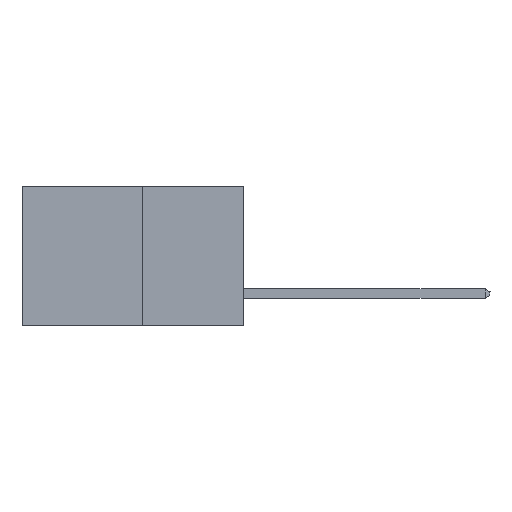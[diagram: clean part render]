
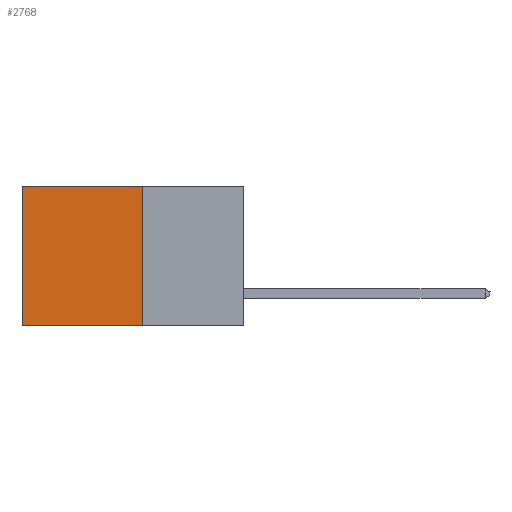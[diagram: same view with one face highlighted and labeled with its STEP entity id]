
A CAD part, left-side view. The second image highlights one B-rep face of the part: STEP entity #2768.
In plain terms, the highlighted planar face has unit normal (-1, 0, 0).
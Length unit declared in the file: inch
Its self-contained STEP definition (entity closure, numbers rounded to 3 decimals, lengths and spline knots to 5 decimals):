
#472 = CARTESIAN_POINT ( 'NONE',  ( 0.277, 0.27, -0.37 ) ) ;
#800 = VERTEX_POINT ( 'NONE', #4747 ) ;
#2022 = EDGE_CURVE ( 'NONE', #10014, #5146, #2332, .T. ) ;
#2332 = LINE ( 'NONE', #14295, #5473 ) ;
#2768 = ADVANCED_FACE ( 'NONE', ( #7432 ), #4299, .F. ) ;
#2903 = EDGE_LOOP ( 'NONE', ( #13023, #15455, #13230, #13313 ) ) ;
#4299 = PLANE ( 'NONE',  #10440 ) ;
#4747 = CARTESIAN_POINT ( 'NONE',  ( 0.277, 0.59, -0.37 ) ) ;
#4897 = VECTOR ( 'NONE', #15755, 39.37008 ) ;
#5146 = VERTEX_POINT ( 'NONE', #472 ) ;
#5473 = VECTOR ( 'NONE', #13830, 39.37008 ) ;
#5757 = DIRECTION ( 'NONE',  ( 0., 1., 0. ) ) ;
#7432 = FACE_OUTER_BOUND ( 'NONE', #2903, .T. ) ;
#7730 = VECTOR ( 'NONE', #16216, 39.37008 ) ;
#9906 = CARTESIAN_POINT ( 'NONE',  ( 0.277, 0.27, 0. ) ) ;
#10014 = VERTEX_POINT ( 'NONE', #14339 ) ;
#10440 = AXIS2_PLACEMENT_3D ( 'NONE', #14002, #14050, #14364 ) ;
#11548 = LINE ( 'NONE', #9906, #4897 ) ;
#12182 = LINE ( 'NONE', #12726, #7730 ) ;
#12311 = VECTOR ( 'NONE', #5757, 39.37008 ) ;
#12726 = CARTESIAN_POINT ( 'NONE',  ( 0.277, 0.59, -0.37 ) ) ;
#13023 = ORIENTED_EDGE ( 'NONE', *, *, #13631, .T. ) ;
#13230 = ORIENTED_EDGE ( 'NONE', *, *, #2022, .F. ) ;
#13313 = ORIENTED_EDGE ( 'NONE', *, *, #15853, .T. ) ;
#13631 = EDGE_CURVE ( 'NONE', #14796, #800, #12182, .T. ) ;
#13830 = DIRECTION ( 'NONE',  ( 0., 0., -1. ) ) ;
#14002 = CARTESIAN_POINT ( 'NONE',  ( 0.277, 0.27, -0.37 ) ) ;
#14050 = DIRECTION ( 'NONE',  ( 1., 0., 0. ) ) ;
#14295 = CARTESIAN_POINT ( 'NONE',  ( 0.277, 0.27, -0.37 ) ) ;
#14339 = CARTESIAN_POINT ( 'NONE',  ( 0.277, 0.27, 0. ) ) ;
#14355 = CARTESIAN_POINT ( 'NONE',  ( 0.277, 0.27, -0.37 ) ) ;
#14364 = DIRECTION ( 'NONE',  ( 0., 0., -1. ) ) ;
#14433 = CARTESIAN_POINT ( 'NONE',  ( 0.277, 0.59, 0. ) ) ;
#14796 = VERTEX_POINT ( 'NONE', #14433 ) ;
#15051 = LINE ( 'NONE', #14355, #12311 ) ;
#15455 = ORIENTED_EDGE ( 'NONE', *, *, #16398, .F. ) ;
#15755 = DIRECTION ( 'NONE',  ( 0., 1., 0. ) ) ;
#15853 = EDGE_CURVE ( 'NONE', #10014, #14796, #11548, .T. ) ;
#16216 = DIRECTION ( 'NONE',  ( 0., 0., -1. ) ) ;
#16398 = EDGE_CURVE ( 'NONE', #5146, #800, #15051, .T. ) ;
